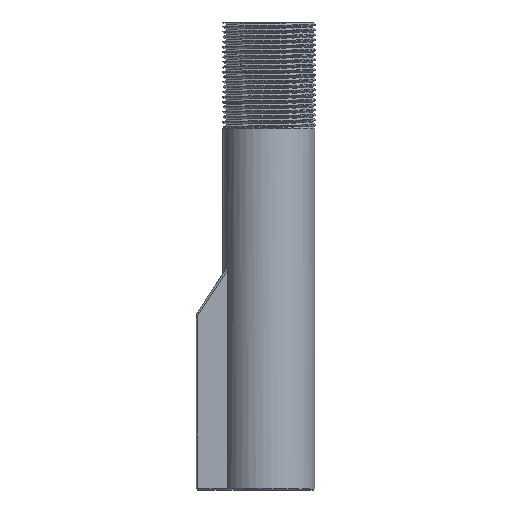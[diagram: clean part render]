
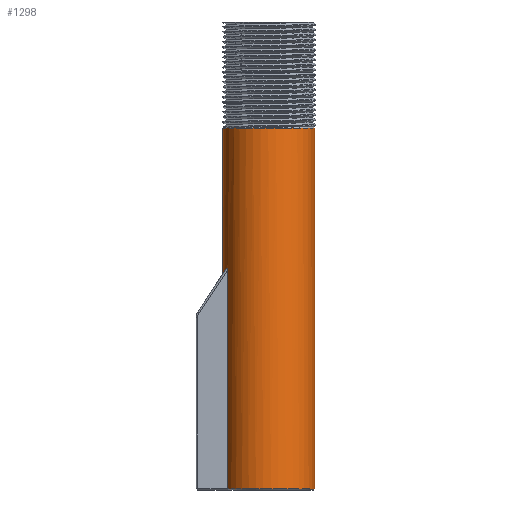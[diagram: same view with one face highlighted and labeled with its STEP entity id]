
A CAD part, front view. The second image highlights one B-rep face of the part: STEP entity #1298.
In plain terms, the highlighted cylindrical face has radius 14.5 mm (diameter 29 mm), a full revolution.
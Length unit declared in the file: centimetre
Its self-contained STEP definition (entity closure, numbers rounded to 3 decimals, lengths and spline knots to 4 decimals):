
#47=LINE($,#1748,#85);
#51=LINE($,#1758,#89);
#85=VECTOR($,#1485,6.9167);
#89=VECTOR($,#1493,6.9167);
#119=ELLIPSE($,#1370,2.6293,1.45);
#131=B_SPLINE_CURVE_WITH_KNOTS($,3,(#1760,#1761,#1762,#1763,#1764,#1765,
#1766,#1767,#1768,#1769,#1770,#1771,#1772,#1773,#1774,#1775),
 .UNSPECIFIED.,.F.,.F.,(4,2,2,2,2,2,2,4),(0.1309,0.1418,
0.1526,0.1619,0.1712,0.1851,
0.199,0.2268),.UNSPECIFIED.);
#132=B_SPLINE_CURVE_WITH_KNOTS($,3,(#1778,#1779,#1780,#1781,#1782,#1783,
#1784,#1785,#1786,#1787,#1788,#1789,#1790,#1791,#1792,#1793),
 .UNSPECIFIED.,.F.,.F.,(4,2,2,2,2,2,2,4),(0.2381,0.2659,
0.2797,0.2936,0.3029,0.3122,0.3231,
0.3339),.UNSPECIFIED.);
#279=CYLINDRICAL_SURFACE($,#1369,1.45);
#295=FACE_BOUND($,#375,.T.);
#314=FACE_OUTER_BOUND($,#374,.T.);
#374=EDGE_LOOP($,(#894,#895,#896,#897,#898,#899));
#375=EDGE_LOOP($,(#900,#901));
#433=CIRCLE($,#1366,1.45);
#435=CIRCLE($,#1371,1.45);
#436=CIRCLE($,#1372,1.45);
#470=VERTEX_POINT($,#1719);
#474=VERTEX_POINT($,#1738);
#475=VERTEX_POINT($,#1747);
#479=VERTEX_POINT($,#1757);
#480=VERTEX_POINT($,#1759);
#481=VERTEX_POINT($,#1776);
#482=VERTEX_POINT($,#1794);
#483=VERTEX_POINT($,#1795);
#653=EDGE_CURVE($,#470,#474,#433,.T.);
#654=EDGE_CURVE($,#474,#475,#47,.T.);
#659=EDGE_CURVE($,#479,#470,#51,.T.);
#660=EDGE_CURVE($,#479,#480,#131,.F.);
#661=EDGE_CURVE($,#481,#480,#119,.T.);
#662=EDGE_CURVE($,#481,#475,#132,.F.);
#663=EDGE_CURVE($,#482,#483,#435,.T.);
#664=EDGE_CURVE($,#483,#482,#436,.T.);
#894=ORIENTED_EDGE($,*,*,#653,.F.);
#895=ORIENTED_EDGE($,*,*,#659,.F.);
#896=ORIENTED_EDGE($,*,*,#660,.T.);
#897=ORIENTED_EDGE($,*,*,#661,.F.);
#898=ORIENTED_EDGE($,*,*,#662,.T.);
#899=ORIENTED_EDGE($,*,*,#654,.F.);
#900=ORIENTED_EDGE($,*,*,#663,.T.);
#901=ORIENTED_EDGE($,*,*,#664,.T.);
#1298=ADVANCED_FACE($,(#314,#295),#279,.T.);
#1366=AXIS2_PLACEMENT_3D($,#1745,#1481,#1482);
#1369=AXIS2_PLACEMENT_3D($,#1756,#1491,#1492);
#1370=AXIS2_PLACEMENT_3D($,#1777,#1494,#1495);
#1371=AXIS2_PLACEMENT_3D($,#1796,#1496,#1497);
#1372=AXIS2_PLACEMENT_3D($,#1797,#1498,#1499);
#1481=DIRECTION('center_axis',(0.,0.,-1.));
#1482=DIRECTION('ref_axis',(0.,1.,0.));
#1485=DIRECTION($,(0.,0.,1.));
#1491=DIRECTION('center_axis',(0.,0.,
1.));
#1492=DIRECTION('ref_axis',(0.,1.,0.));
#1493=DIRECTION($,(0.,0.,-1.));
#1494=DIRECTION('center_axis',(0.834,0.,
-0.551));
#1495=DIRECTION('ref_axis',(-0.551,0.,-0.834));
#1496=DIRECTION('center_axis',(0.,0.,-1.));
#1497=DIRECTION('ref_axis',(0.,1.,0.));
#1498=DIRECTION('center_axis',(0.,0.,-1.));
#1499=DIRECTION('ref_axis',(0.,1.,0.));
#1719=CARTESIAN_POINT('',(-4.3222,9.625,2.04));
#1738=CARTESIAN_POINT('',(-4.3222,8.375,2.04));
#1745=CARTESIAN_POINT('Origin',(-3.0139,9.,2.04));
#1747=CARTESIAN_POINT('',(-4.3222,8.375,8.9567));
#1748=CARTESIAN_POINT($,(-4.3222,8.375,9.5474));
#1756=CARTESIAN_POINT('Origin',(-3.0139,9.,9.5474));
#1757=CARTESIAN_POINT('',(-4.3222,9.625,8.9567));
#1758=CARTESIAN_POINT($,(-4.3222,9.625,9.5474));
#1759=CARTESIAN_POINT('',(-4.345,9.575,9.013));
#1760=CARTESIAN_POINT('Ctrl Pts',(-4.345,9.575,9.013));
#1761=CARTESIAN_POINT('Ctrl Pts',(-4.3437,9.5778,9.0149));
#1762=CARTESIAN_POINT('Ctrl Pts',(-4.3423,9.5811,9.0166));
#1763=CARTESIAN_POINT('Ctrl Pts',(-4.3393,9.588,9.0187));
#1764=CARTESIAN_POINT('Ctrl Pts',(-4.3377,9.5915,9.0191));
#1765=CARTESIAN_POINT('Ctrl Pts',(-4.335,9.5976,9.0185));
#1766=CARTESIAN_POINT('Ctrl Pts',(-4.3336,9.6006,9.0176));
#1767=CARTESIAN_POINT('Ctrl Pts',(-4.3312,9.6059,9.0147));
#1768=CARTESIAN_POINT('Ctrl Pts',(-4.3301,9.6084,9.0126));
#1769=CARTESIAN_POINT('Ctrl Pts',(-4.3278,9.6133,9.0071));
#1770=CARTESIAN_POINT('Ctrl Pts',(-4.3267,9.6156,9.0032));
#1771=CARTESIAN_POINT('Ctrl Pts',(-4.3249,9.6194,8.9948));
#1772=CARTESIAN_POINT('Ctrl Pts',(-4.3242,9.6209,8.9903));
#1773=CARTESIAN_POINT('Ctrl Pts',(-4.3226,9.6242,8.9761));
#1774=CARTESIAN_POINT('Ctrl Pts',(-4.3222,9.625,8.966));
#1775=CARTESIAN_POINT('Ctrl Pts',(-4.3222,9.625,8.9567));
#1776=CARTESIAN_POINT('',(-4.345,8.425,9.013));
#1777=CARTESIAN_POINT('Origin',(-3.0139,9.,11.0266));
#1778=CARTESIAN_POINT('Ctrl Pts',(-4.3222,8.375,8.9567));
#1779=CARTESIAN_POINT('Ctrl Pts',(-4.3222,8.375,8.966));
#1780=CARTESIAN_POINT('Ctrl Pts',(-4.3226,8.3758,8.9761));
#1781=CARTESIAN_POINT('Ctrl Pts',(-4.3242,8.3791,8.9903));
#1782=CARTESIAN_POINT('Ctrl Pts',(-4.3249,8.3806,8.9948));
#1783=CARTESIAN_POINT('Ctrl Pts',(-4.3267,8.3844,9.0032));
#1784=CARTESIAN_POINT('Ctrl Pts',(-4.3278,8.3867,9.0071));
#1785=CARTESIAN_POINT('Ctrl Pts',(-4.3301,8.3916,9.0126));
#1786=CARTESIAN_POINT('Ctrl Pts',(-4.3312,8.3941,9.0147));
#1787=CARTESIAN_POINT('Ctrl Pts',(-4.3336,8.3994,9.0176));
#1788=CARTESIAN_POINT('Ctrl Pts',(-4.335,8.4024,9.0185));
#1789=CARTESIAN_POINT('Ctrl Pts',(-4.3377,8.4085,9.0191));
#1790=CARTESIAN_POINT('Ctrl Pts',(-4.3393,8.412,9.0187));
#1791=CARTESIAN_POINT('Ctrl Pts',(-4.3423,8.4189,9.0166));
#1792=CARTESIAN_POINT('Ctrl Pts',(-4.3437,8.4222,9.0149));
#1793=CARTESIAN_POINT('Ctrl Pts',(-4.345,8.425,9.013));
#1794=CARTESIAN_POINT('',(-2.2092,10.2063,13.4474));
#1795=CARTESIAN_POINT('',(-4.3904,9.4557,13.4474));
#1796=CARTESIAN_POINT('Origin',(-3.0139,9.,13.4474));
#1797=CARTESIAN_POINT('Origin',(-3.0139,9.,13.4474));
